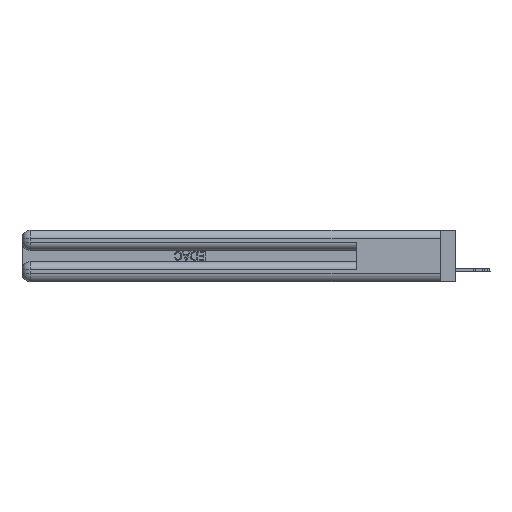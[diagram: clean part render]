
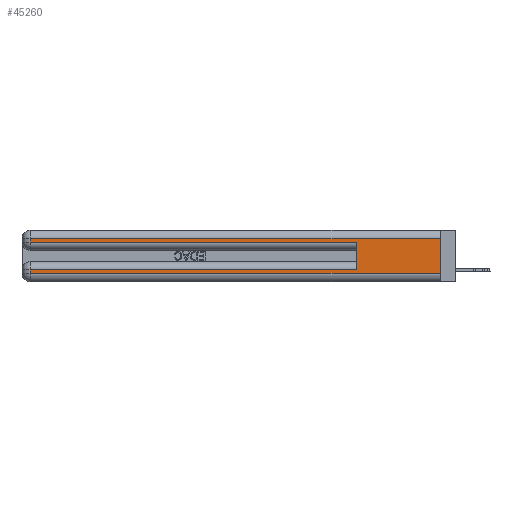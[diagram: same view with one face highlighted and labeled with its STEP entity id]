
A CAD part, left-side view. The second image highlights one B-rep face of the part: STEP entity #45260.
In plain terms, the highlighted planar face has unit normal (-1, 0, 0).
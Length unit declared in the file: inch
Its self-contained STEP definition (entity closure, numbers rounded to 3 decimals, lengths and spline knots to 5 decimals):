
#1848 = VECTOR ( 'NONE', #25183, 39.37008 ) ;
#2109 = VERTEX_POINT ( 'NONE', #45498 ) ;
#2479 = CARTESIAN_POINT ( 'NONE',  ( 0., 0.6, 0.085 ) ) ;
#2614 = CARTESIAN_POINT ( 'NONE',  ( 0., 0., 0.085 ) ) ;
#3711 = VERTEX_POINT ( 'NONE', #31902 ) ;
#4461 = CARTESIAN_POINT ( 'NONE',  ( 0., 0., 0.31 ) ) ;
#6205 = CARTESIAN_POINT ( 'NONE',  ( 0., 2.94, 0.06 ) ) ;
#6571 = EDGE_CURVE ( 'NONE', #10098, #45936, #52619, .T. ) ;
#6952 = PLANE ( 'NONE',  #21635 ) ;
#9167 = EDGE_CURVE ( 'NONE', #50678, #3711, #39496, .T. ) ;
#10098 = VERTEX_POINT ( 'NONE', #6205 ) ;
#11486 = EDGE_CURVE ( 'NONE', #24291, #14074, #14445, .T. ) ;
#11679 = CARTESIAN_POINT ( 'NONE',  ( 0., 2.94, 0.37 ) ) ;
#11942 = DIRECTION ( 'NONE',  ( 0., 0., -1. ) ) ;
#12065 = CARTESIAN_POINT ( 'NONE',  ( 0., 0., 0.285 ) ) ;
#13544 = CARTESIAN_POINT ( 'NONE',  ( 0., 2.94, 0.085 ) ) ;
#13703 = EDGE_CURVE ( 'NONE', #14074, #10098, #24708, .T. ) ;
#14074 = VERTEX_POINT ( 'NONE', #13544 ) ;
#14445 = LINE ( 'NONE', #2614, #30776 ) ;
#14622 = DIRECTION ( 'NONE',  ( 0., -1., 0. ) ) ;
#15130 = CARTESIAN_POINT ( 'NONE',  ( 0., 2.94, 0.37 ) ) ;
#18071 = EDGE_LOOP ( 'NONE', ( #40945, #29729, #20476, #20726, #34144, #21666, #39447, #29520 ) ) ;
#18090 = CARTESIAN_POINT ( 'NONE',  ( 0., 0., 0.06 ) ) ;
#18787 = CARTESIAN_POINT ( 'NONE',  ( 0., 0., 0.37 ) ) ;
#20053 = VERTEX_POINT ( 'NONE', #33518 ) ;
#20476 = ORIENTED_EDGE ( 'NONE', *, *, #9167, .T. ) ;
#20726 = ORIENTED_EDGE ( 'NONE', *, *, #43271, .T. ) ;
#20955 = DIRECTION ( 'NONE',  ( 0., 1., 0. ) ) ;
#21635 = AXIS2_PLACEMENT_3D ( 'NONE', #24548, #36636, #11942 ) ;
#21666 = ORIENTED_EDGE ( 'NONE', *, *, #11486, .T. ) ;
#21753 = VECTOR ( 'NONE', #39596, 39.37008 ) ;
#22268 = CARTESIAN_POINT ( 'NONE',  ( 0., 2.94, 0.31 ) ) ;
#22348 = VECTOR ( 'NONE', #25712, 39.37008 ) ;
#24291 = VERTEX_POINT ( 'NONE', #2479 ) ;
#24548 = CARTESIAN_POINT ( 'NONE',  ( 0., 0., 0.37 ) ) ;
#24708 = LINE ( 'NONE', #15130, #44284 ) ;
#25183 = DIRECTION ( 'NONE',  ( 0., -1., 0. ) ) ;
#25712 = DIRECTION ( 'NONE',  ( 0., 0., 1. ) ) ;
#29520 = ORIENTED_EDGE ( 'NONE', *, *, #6571, .T. ) ;
#29729 = ORIENTED_EDGE ( 'NONE', *, *, #38706, .T. ) ;
#30776 = VECTOR ( 'NONE', #43754, 39.37008 ) ;
#31902 = CARTESIAN_POINT ( 'NONE',  ( 0., 2.94, 0.285 ) ) ;
#31954 = DIRECTION ( 'NONE',  ( 0., 0., -1. ) ) ;
#32464 = VECTOR ( 'NONE', #14622, 39.37008 ) ;
#33518 = CARTESIAN_POINT ( 'NONE',  ( 0., 0.6, 0.285 ) ) ;
#33798 = FACE_OUTER_BOUND ( 'NONE', #18071, .T. ) ;
#34144 = ORIENTED_EDGE ( 'NONE', *, *, #41588, .F. ) ;
#34624 = LINE ( 'NONE', #12065, #1848 ) ;
#36191 = DIRECTION ( 'NONE',  ( 0., 0., -1. ) ) ;
#36636 = DIRECTION ( 'NONE',  ( 1., 0., 0. ) ) ;
#38706 = EDGE_CURVE ( 'NONE', #2109, #50678, #44627, .T. ) ;
#39447 = ORIENTED_EDGE ( 'NONE', *, *, #13703, .T. ) ;
#39496 = LINE ( 'NONE', #11679, #52528 ) ;
#39596 = DIRECTION ( 'NONE',  ( 0., 0., -1. ) ) ;
#40945 = ORIENTED_EDGE ( 'NONE', *, *, #47407, .F. ) ;
#41588 = EDGE_CURVE ( 'NONE', #24291, #20053, #53836, .T. ) ;
#42195 = CARTESIAN_POINT ( 'NONE',  ( 0., 0.6, 0.145 ) ) ;
#43271 = EDGE_CURVE ( 'NONE', #3711, #20053, #34624, .T. ) ;
#43754 = DIRECTION ( 'NONE',  ( 0., 1., 0. ) ) ;
#44284 = VECTOR ( 'NONE', #31954, 39.37008 ) ;
#44627 = LINE ( 'NONE', #4461, #45931 ) ;
#44953 = CARTESIAN_POINT ( 'NONE',  ( 0., 0., 0.06 ) ) ;
#45260 = ADVANCED_FACE ( 'NONE', ( #33798 ), #6952, .F. ) ;
#45498 = CARTESIAN_POINT ( 'NONE',  ( 0., 0., 0.31 ) ) ;
#45931 = VECTOR ( 'NONE', #20955, 39.37008 ) ;
#45936 = VERTEX_POINT ( 'NONE', #44953 ) ;
#45982 = LINE ( 'NONE', #18787, #21753 ) ;
#47407 = EDGE_CURVE ( 'NONE', #2109, #45936, #45982, .T. ) ;
#50678 = VERTEX_POINT ( 'NONE', #22268 ) ;
#52528 = VECTOR ( 'NONE', #36191, 39.37008 ) ;
#52619 = LINE ( 'NONE', #18090, #32464 ) ;
#53836 = LINE ( 'NONE', #42195, #22348 ) ;
